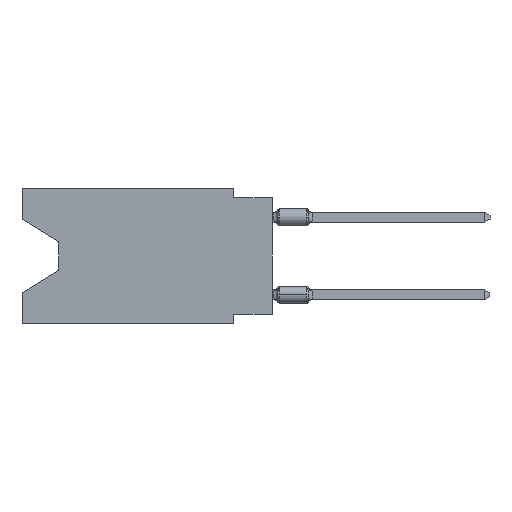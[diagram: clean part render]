
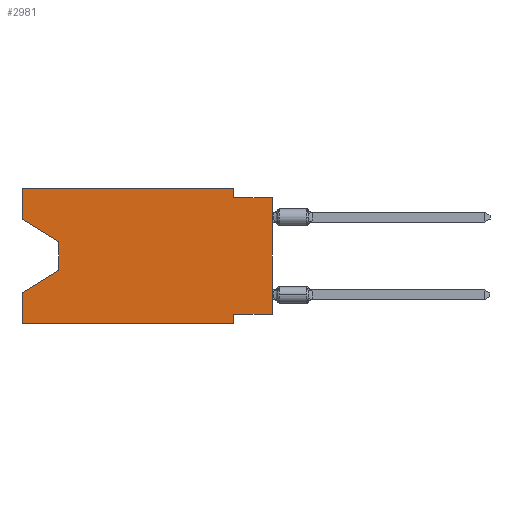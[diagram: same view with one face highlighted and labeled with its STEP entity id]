
A CAD part, left-side view. The second image highlights one B-rep face of the part: STEP entity #2981.
In plain terms, the highlighted planar face has unit normal (-1, 0, 0).
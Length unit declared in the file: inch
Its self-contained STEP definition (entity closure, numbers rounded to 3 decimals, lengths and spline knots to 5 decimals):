
#280 = ORIENTED_EDGE ( 'NONE', *, *, #19821, .T. ) ;
#757 = ORIENTED_EDGE ( 'NONE', *, *, #18083, .T. ) ;
#1013 = LINE ( 'NONE', #22276, #2768 ) ;
#1144 = CARTESIAN_POINT ( 'NONE',  ( 0., 0., -0.325 ) ) ;
#1488 = DIRECTION ( 'NONE',  ( 0., 0., -1. ) ) ;
#1679 = DIRECTION ( 'NONE',  ( 0., -1., 0. ) ) ;
#1887 = LINE ( 'NONE', #25152, #3150 ) ;
#2258 = VERTEX_POINT ( 'NONE', #15159 ) ;
#2424 = CARTESIAN_POINT ( 'NONE',  ( 0., 0.55, -0.138 ) ) ;
#2485 = CARTESIAN_POINT ( 'NONE',  ( 0., 0., 0. ) ) ;
#2768 = VECTOR ( 'NONE', #20177, 39.37008 ) ;
#2981 = ADVANCED_FACE ( 'NONE', ( #27881 ), #10659, .F. ) ;
#3121 = LINE ( 'NONE', #1144, #7688 ) ;
#3150 = VECTOR ( 'NONE', #14968, 39.37008 ) ;
#3236 = ORIENTED_EDGE ( 'NONE', *, *, #4513, .F. ) ;
#3261 = CARTESIAN_POINT ( 'NONE',  ( 0., 0.645, -0.35 ) ) ;
#3322 = VECTOR ( 'NONE', #27871, 39.37008 ) ;
#3723 = CARTESIAN_POINT ( 'NONE',  ( 0., 0.645, -0.08025 ) ) ;
#3740 = ORIENTED_EDGE ( 'NONE', *, *, #10881, .F. ) ;
#3810 = LINE ( 'NONE', #3261, #17182 ) ;
#3962 = CARTESIAN_POINT ( 'NONE',  ( 0., 0.55, -0.212 ) ) ;
#4428 = CARTESIAN_POINT ( 'NONE',  ( 0., 0.1, -0.025 ) ) ;
#4513 = EDGE_CURVE ( 'NONE', #16407, #15229, #10377, .T. ) ;
#4693 = DIRECTION ( 'NONE',  ( 0., 0.855, -0.519 ) ) ;
#4943 = CARTESIAN_POINT ( 'NONE',  ( 0., 0.645, -0.08025 ) ) ;
#6451 = LINE ( 'NONE', #25343, #3322 ) ;
#7079 = DIRECTION ( 'NONE',  ( 0., 1., 0. ) ) ;
#7143 = LINE ( 'NONE', #24336, #15668 ) ;
#7438 = EDGE_CURVE ( 'NONE', #27849, #17721, #7143, .T. ) ;
#7688 = VECTOR ( 'NONE', #7079, 39.37008 ) ;
#8321 = ORIENTED_EDGE ( 'NONE', *, *, #23982, .F. ) ;
#8326 = EDGE_CURVE ( 'NONE', #12629, #10625, #13255, .T. ) ;
#8550 = ORIENTED_EDGE ( 'NONE', *, *, #8326, .T. ) ;
#8778 = CARTESIAN_POINT ( 'NONE',  ( 0., 0.1, 0. ) ) ;
#9040 = CARTESIAN_POINT ( 'NONE',  ( 0., 0.645, -0.26975 ) ) ;
#9897 = VECTOR ( 'NONE', #26935, 39.37008 ) ;
#10377 = LINE ( 'NONE', #24903, #23914 ) ;
#10515 = EDGE_CURVE ( 'NONE', #14339, #2258, #17120, .T. ) ;
#10592 = CARTESIAN_POINT ( 'NONE',  ( 0., 0.1, -0.325 ) ) ;
#10625 = VERTEX_POINT ( 'NONE', #9040 ) ;
#10659 = PLANE ( 'NONE',  #25226 ) ;
#10699 = ORIENTED_EDGE ( 'NONE', *, *, #10515, .T. ) ;
#10881 = EDGE_CURVE ( 'NONE', #15936, #2258, #18452, .T. ) ;
#11821 = CARTESIAN_POINT ( 'NONE',  ( 0., 0.645, 0. ) ) ;
#12629 = VERTEX_POINT ( 'NONE', #3962 ) ;
#13255 = LINE ( 'NONE', #26123, #20211 ) ;
#13791 = CARTESIAN_POINT ( 'NONE',  ( 0., 0.1, -0.35 ) ) ;
#13934 = DIRECTION ( 'NONE',  ( 0., 0., 1. ) ) ;
#14339 = VERTEX_POINT ( 'NONE', #14489 ) ;
#14489 = CARTESIAN_POINT ( 'NONE',  ( 0., 0., -0.325 ) ) ;
#14968 = DIRECTION ( 'NONE',  ( 0., 0., -1. ) ) ;
#15100 = VERTEX_POINT ( 'NONE', #2424 ) ;
#15156 = DIRECTION ( 'NONE',  ( 0., 0., -1. ) ) ;
#15159 = CARTESIAN_POINT ( 'NONE',  ( 0., 0., -0.025 ) ) ;
#15229 = VERTEX_POINT ( 'NONE', #13791 ) ;
#15614 = DIRECTION ( 'NONE',  ( 0., -0.855, -0.519 ) ) ;
#15668 = VECTOR ( 'NONE', #22193, 39.37008 ) ;
#15936 = VERTEX_POINT ( 'NONE', #4428 ) ;
#16217 = VECTOR ( 'NONE', #15614, 39.37008 ) ;
#16407 = VERTEX_POINT ( 'NONE', #10592 ) ;
#17120 = LINE ( 'NONE', #2485, #24736 ) ;
#17182 = VECTOR ( 'NONE', #1679, 39.37008 ) ;
#17449 = EDGE_CURVE ( 'NONE', #17721, #15936, #1887, .T. ) ;
#17721 = VERTEX_POINT ( 'NONE', #8778 ) ;
#18083 = EDGE_CURVE ( 'NONE', #27691, #15100, #20548, .T. ) ;
#18120 = EDGE_CURVE ( 'NONE', #27691, #27849, #24662, .T. ) ;
#18452 = LINE ( 'NONE', #24955, #9897 ) ;
#18506 = EDGE_CURVE ( 'NONE', #14339, #16407, #3121, .T. ) ;
#19251 = DIRECTION ( 'NONE',  ( 1., 0., 0. ) ) ;
#19711 = ORIENTED_EDGE ( 'NONE', *, *, #18506, .F. ) ;
#19821 = EDGE_CURVE ( 'NONE', #15100, #12629, #1013, .T. ) ;
#19895 = ORIENTED_EDGE ( 'NONE', *, *, #17449, .F. ) ;
#20074 = DIRECTION ( 'NONE',  ( 0., 0., 1. ) ) ;
#20177 = DIRECTION ( 'NONE',  ( 0., 0., -1. ) ) ;
#20211 = VECTOR ( 'NONE', #4693, 39.37008 ) ;
#20278 = CARTESIAN_POINT ( 'NONE',  ( 0., 0.645, 0. ) ) ;
#20548 = LINE ( 'NONE', #4943, #16217 ) ;
#20665 = EDGE_CURVE ( 'NONE', #22877, #15229, #3810, .T. ) ;
#21160 = VECTOR ( 'NONE', #13934, 39.37008 ) ;
#21351 = CARTESIAN_POINT ( 'NONE',  ( 0., 0.645, -0.35 ) ) ;
#21649 = CARTESIAN_POINT ( 'NONE',  ( 0., 0.645, 0. ) ) ;
#22193 = DIRECTION ( 'NONE',  ( 0., -1., 0. ) ) ;
#22276 = CARTESIAN_POINT ( 'NONE',  ( 0., 0.55, -0.138 ) ) ;
#22877 = VERTEX_POINT ( 'NONE', #21351 ) ;
#23914 = VECTOR ( 'NONE', #1488, 39.37008 ) ;
#23982 = EDGE_CURVE ( 'NONE', #22877, #10625, #6451, .T. ) ;
#24336 = CARTESIAN_POINT ( 'NONE',  ( 0., 0.645, 0. ) ) ;
#24662 = LINE ( 'NONE', #11821, #21160 ) ;
#24736 = VECTOR ( 'NONE', #20074, 39.37008 ) ;
#24901 = ORIENTED_EDGE ( 'NONE', *, *, #20665, .T. ) ;
#24903 = CARTESIAN_POINT ( 'NONE',  ( 0., 0.1, -0.35 ) ) ;
#24955 = CARTESIAN_POINT ( 'NONE',  ( 0., 0., -0.025 ) ) ;
#25027 = ORIENTED_EDGE ( 'NONE', *, *, #18120, .F. ) ;
#25152 = CARTESIAN_POINT ( 'NONE',  ( 0., 0.1, 0. ) ) ;
#25226 = AXIS2_PLACEMENT_3D ( 'NONE', #21649, #19251, #15156 ) ;
#25343 = CARTESIAN_POINT ( 'NONE',  ( 0., 0.645, 0. ) ) ;
#26123 = CARTESIAN_POINT ( 'NONE',  ( 0., 0.55, -0.212 ) ) ;
#26231 = ORIENTED_EDGE ( 'NONE', *, *, #7438, .F. ) ;
#26935 = DIRECTION ( 'NONE',  ( 0., -1., 0. ) ) ;
#27362 = EDGE_LOOP ( 'NONE', ( #757, #280, #8550, #8321, #24901, #3236, #19711, #10699, #3740, #19895, #26231, #25027 ) ) ;
#27691 = VERTEX_POINT ( 'NONE', #3723 ) ;
#27849 = VERTEX_POINT ( 'NONE', #20278 ) ;
#27871 = DIRECTION ( 'NONE',  ( 0., 0., 1. ) ) ;
#27881 = FACE_OUTER_BOUND ( 'NONE', #27362, .T. ) ;
